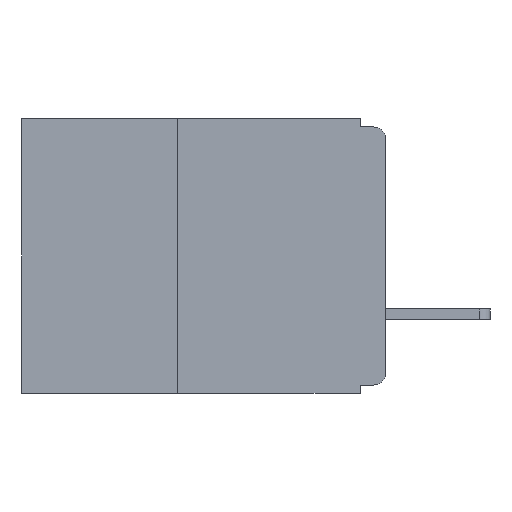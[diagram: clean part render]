
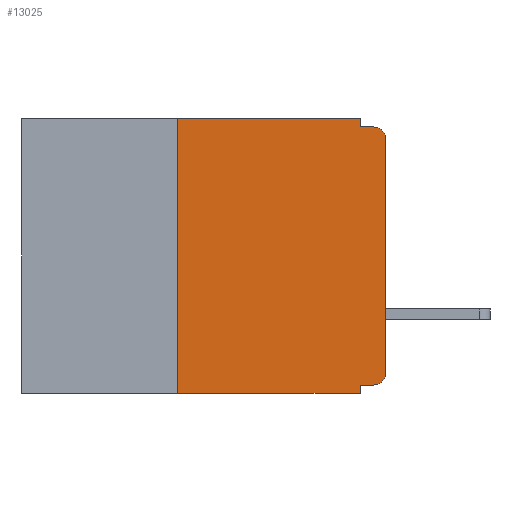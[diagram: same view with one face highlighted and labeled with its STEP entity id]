
A CAD part, left-side view. The second image highlights one B-rep face of the part: STEP entity #13025.
In plain terms, the highlighted planar face has unit normal (-1, 0, 0).
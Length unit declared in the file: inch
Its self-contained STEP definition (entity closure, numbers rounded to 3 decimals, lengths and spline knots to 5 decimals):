
#650 = CARTESIAN_POINT ( 'NONE',  ( 0., 0.031, -0.01 ) ) ;
#733 = VERTEX_POINT ( 'NONE', #20992 ) ;
#804 = CARTESIAN_POINT ( 'NONE',  ( 0., 0.015, -0.32 ) ) ;
#1154 = VERTEX_POINT ( 'NONE', #8248 ) ;
#1200 = CARTESIAN_POINT ( 'NONE',  ( 0., 0.437, 0. ) ) ;
#1486 = EDGE_LOOP ( 'NONE', ( #22141, #21958, #17445, #22590, #2556, #9592, #25180, #23391, #21250, #23459 ) ) ;
#1822 = CARTESIAN_POINT ( 'NONE',  ( 0., 0.25, 0. ) ) ;
#1892 = CARTESIAN_POINT ( 'NONE',  ( 0., 0.437, -0.33 ) ) ;
#1910 = DIRECTION ( 'NONE',  ( 0., 1., 0. ) ) ;
#2379 = VECTOR ( 'NONE', #11849, 39.37008 ) ;
#2556 = ORIENTED_EDGE ( 'NONE', *, *, #18790, .F. ) ;
#2633 = EDGE_CURVE ( 'NONE', #17553, #11827, #15477, .T. ) ;
#3719 = CARTESIAN_POINT ( 'NONE',  ( 0., 0.015, -0.025 ) ) ;
#3740 = EDGE_CURVE ( 'NONE', #1154, #23065, #22854, .T. ) ;
#4092 = VECTOR ( 'NONE', #11068, 39.37008 ) ;
#5668 = FACE_OUTER_BOUND ( 'NONE', #1486, .T. ) ;
#5714 = DIRECTION ( 'NONE',  ( 0., 0., -1. ) ) ;
#5836 = DIRECTION ( 'NONE',  ( 1., 0., 0. ) ) ;
#6099 = VECTOR ( 'NONE', #1910, 39.37008 ) ;
#6113 = AXIS2_PLACEMENT_3D ( 'NONE', #17712, #5836, #19717 ) ;
#6475 = CIRCLE ( 'NONE', #16778, 0.015 ) ;
#6559 = EDGE_CURVE ( 'NONE', #733, #23065, #7614, .T. ) ;
#6725 = LINE ( 'NONE', #9705, #6099 ) ;
#6980 = EDGE_CURVE ( 'NONE', #11827, #13832, #18766, .T. ) ;
#7614 = LINE ( 'NONE', #1892, #2379 ) ;
#8152 = DIRECTION ( 'NONE',  ( -1., 0., 0. ) ) ;
#8248 = CARTESIAN_POINT ( 'NONE',  ( 0., 0.031, -0.32 ) ) ;
#8480 = LINE ( 'NONE', #8689, #17772 ) ;
#8689 = CARTESIAN_POINT ( 'NONE',  ( 0., 0.031, 0. ) ) ;
#9426 = LINE ( 'NONE', #1200, #4092 ) ;
#9592 = ORIENTED_EDGE ( 'NONE', *, *, #25412, .F. ) ;
#9705 = CARTESIAN_POINT ( 'NONE',  ( 0., 0., -0.32 ) ) ;
#9912 = VECTOR ( 'NONE', #20795, 39.37008 ) ;
#10524 = LINE ( 'NONE', #22758, #9912 ) ;
#10719 = DIRECTION ( 'NONE',  ( 0., 0., -1. ) ) ;
#11068 = DIRECTION ( 'NONE',  ( 0., -1., 0. ) ) ;
#11710 = LINE ( 'NONE', #18786, #16302 ) ;
#11827 = VERTEX_POINT ( 'NONE', #15380 ) ;
#11849 = DIRECTION ( 'NONE',  ( 0., -1., 0. ) ) ;
#12517 = CARTESIAN_POINT ( 'NONE',  ( 0., 0.015, -0.01 ) ) ;
#12669 = VERTEX_POINT ( 'NONE', #804 ) ;
#13025 = ADVANCED_FACE ( 'NONE', ( #5668 ), #17631, .F. ) ;
#13381 = CARTESIAN_POINT ( 'NONE',  ( 0., 0., -0.305 ) ) ;
#13632 = AXIS2_PLACEMENT_3D ( 'NONE', #3719, #17595, #5714 ) ;
#13792 = DIRECTION ( 'NONE',  ( 0., 0., -1. ) ) ;
#13832 = VERTEX_POINT ( 'NONE', #12517 ) ;
#14404 = CARTESIAN_POINT ( 'NONE',  ( 0., 0.031, -0.33 ) ) ;
#15362 = EDGE_CURVE ( 'NONE', #12669, #17553, #6475, .T. ) ;
#15380 = CARTESIAN_POINT ( 'NONE',  ( 0., 0., -0.025 ) ) ;
#15477 = LINE ( 'NONE', #24234, #24730 ) ;
#16302 = VECTOR ( 'NONE', #20789, 39.37008 ) ;
#16503 = VERTEX_POINT ( 'NONE', #1822 ) ;
#16545 = EDGE_CURVE ( 'NONE', #12669, #1154, #6725, .T. ) ;
#16778 = AXIS2_PLACEMENT_3D ( 'NONE', #20033, #8152, #22016 ) ;
#17445 = ORIENTED_EDGE ( 'NONE', *, *, #21319, .F. ) ;
#17553 = VERTEX_POINT ( 'NONE', #13381 ) ;
#17595 = DIRECTION ( 'NONE',  ( -1., 0., 0. ) ) ;
#17597 = VECTOR ( 'NONE', #13792, 39.37008 ) ;
#17631 = PLANE ( 'NONE',  #6113 ) ;
#17712 = CARTESIAN_POINT ( 'NONE',  ( 0., 0.437, 0. ) ) ;
#17772 = VECTOR ( 'NONE', #10719, 39.37008 ) ;
#18441 = CARTESIAN_POINT ( 'NONE',  ( 0., 0.031, 0. ) ) ;
#18634 = EDGE_CURVE ( 'NONE', #22886, #21191, #8480, .T. ) ;
#18766 = CIRCLE ( 'NONE', #13632, 0.015 ) ;
#18786 = CARTESIAN_POINT ( 'NONE',  ( 0., 0.25, -0.33 ) ) ;
#18790 = EDGE_CURVE ( 'NONE', #16503, #22886, #9426, .T. ) ;
#19056 = CARTESIAN_POINT ( 'NONE',  ( 0., 0.031, -0.33 ) ) ;
#19717 = DIRECTION ( 'NONE',  ( 0., 0., -1. ) ) ;
#20033 = CARTESIAN_POINT ( 'NONE',  ( 0., 0.015, -0.305 ) ) ;
#20789 = DIRECTION ( 'NONE',  ( 0., 0., 1. ) ) ;
#20795 = DIRECTION ( 'NONE',  ( 0., -1., 0. ) ) ;
#20992 = CARTESIAN_POINT ( 'NONE',  ( 0., 0.25, -0.33 ) ) ;
#21191 = VERTEX_POINT ( 'NONE', #650 ) ;
#21250 = ORIENTED_EDGE ( 'NONE', *, *, #16545, .F. ) ;
#21319 = EDGE_CURVE ( 'NONE', #21191, #13832, #10524, .T. ) ;
#21958 = ORIENTED_EDGE ( 'NONE', *, *, #6980, .T. ) ;
#22016 = DIRECTION ( 'NONE',  ( 0., 0., -1. ) ) ;
#22141 = ORIENTED_EDGE ( 'NONE', *, *, #2633, .T. ) ;
#22590 = ORIENTED_EDGE ( 'NONE', *, *, #18634, .F. ) ;
#22758 = CARTESIAN_POINT ( 'NONE',  ( 0., 0., -0.01 ) ) ;
#22854 = LINE ( 'NONE', #14404, #17597 ) ;
#22886 = VERTEX_POINT ( 'NONE', #18441 ) ;
#23065 = VERTEX_POINT ( 'NONE', #19056 ) ;
#23391 = ORIENTED_EDGE ( 'NONE', *, *, #3740, .F. ) ;
#23459 = ORIENTED_EDGE ( 'NONE', *, *, #15362, .T. ) ;
#24214 = DIRECTION ( 'NONE',  ( 0., 0., 1. ) ) ;
#24234 = CARTESIAN_POINT ( 'NONE',  ( 0., 0., 0. ) ) ;
#24730 = VECTOR ( 'NONE', #24214, 39.37008 ) ;
#25180 = ORIENTED_EDGE ( 'NONE', *, *, #6559, .T. ) ;
#25412 = EDGE_CURVE ( 'NONE', #733, #16503, #11710, .T. ) ;
